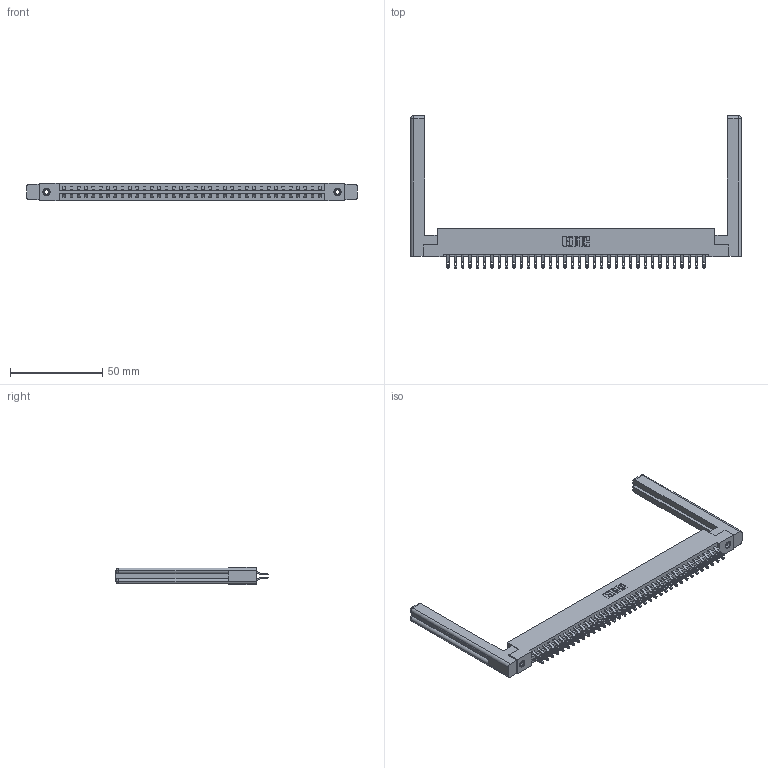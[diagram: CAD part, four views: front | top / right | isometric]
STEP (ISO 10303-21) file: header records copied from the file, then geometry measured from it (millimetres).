
FILE_DESCRIPTION (( 'STEP AP203' ), '1' );
FILE_NAME ('387-072-555-258.STEP', '2019-10-22T00:23:21', ( '' ), ( '' ), 'SwSTEP 2.0', 'SolidWorks 2016', '' );
FILE_SCHEMA (( 'CONFIG_CONTROL_DESIGN' ));
Length unit declared in the file: inch
Products named in the file (5): 345-292-001_555 Tail; 387-072-555-258; 307-220-058; 345-250-001_345-250-001-102; 337 Part_Flush Mounting Lugs - 0.156 Dia-TI
Assembly tree (77 placements, depth 2):
  387-072-555-258
    337 Part_Flush Mounting Lugs - 0.156 Dia-TI
    345-292-001_555 Tail  x72
    345-250-001_345-250-001-102  x2
    307-220-058  x2
Bounding box: 179.27 x 82.56 x 9.4 mm (x, y, z)
Volume: 26164.6 mm3; surface area: 27280.1 mm2
Topology: 77 solids, 77 shells, 4576 faces, 14273 edges, 9502 vertices
Faces by surface type: plane 2746, cylinder 1806, cone 12, torus 12
Entity records: 31648 total; most frequent: CARTESIAN_POINT 5379, ORIENTED_EDGE 5224, DIRECTION 4572, EDGE_CURVE 2612, VECTOR 2416, LINE 2416, VERTEX_POINT 1734, AXIS2_PLACEMENT_3D 1078
